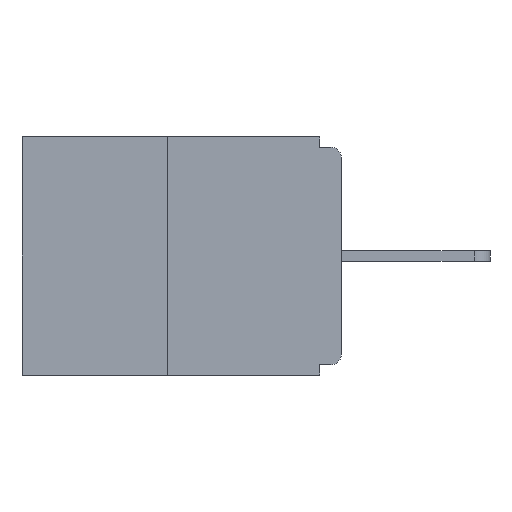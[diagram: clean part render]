
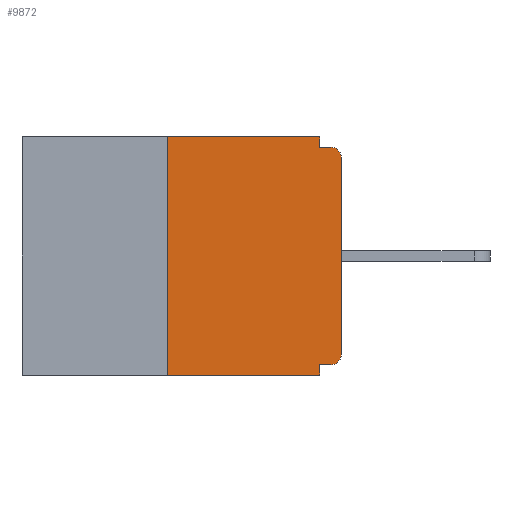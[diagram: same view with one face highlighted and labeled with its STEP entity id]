
A CAD part, left-side view. The second image highlights one B-rep face of the part: STEP entity #9872.
In plain terms, the highlighted planar face has unit normal (-1, 0, 0).
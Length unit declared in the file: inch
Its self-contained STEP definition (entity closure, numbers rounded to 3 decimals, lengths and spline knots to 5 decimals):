
#187 = ORIENTED_EDGE ( 'NONE', *, *, #12590, .F. ) ;
#594 = DIRECTION ( 'NONE',  ( -1., 0., 0. ) ) ;
#603 = CARTESIAN_POINT ( 'NONE',  ( 0., 0.46, -0.343 ) ) ;
#630 = VERTEX_POINT ( 'NONE', #15528 ) ;
#683 = CARTESIAN_POINT ( 'NONE',  ( 0., 0., -0.328 ) ) ;
#1034 = EDGE_CURVE ( 'NONE', #630, #7725, #15452, .T. ) ;
#1348 = VERTEX_POINT ( 'NONE', #3470 ) ;
#1537 = CARTESIAN_POINT ( 'NONE',  ( 0., 0.46, 0. ) ) ;
#1681 = CIRCLE ( 'NONE', #7419, 0.015 ) ;
#1764 = DIRECTION ( 'NONE',  ( 1., 0., 0. ) ) ;
#2621 = ORIENTED_EDGE ( 'NONE', *, *, #1034, .F. ) ;
#3470 = CARTESIAN_POINT ( 'NONE',  ( 0., 0.031, -0.328 ) ) ;
#3579 = EDGE_CURVE ( 'NONE', #10144, #4300, #1681, .T. ) ;
#3772 = CARTESIAN_POINT ( 'NONE',  ( 0., 0.031, 0. ) ) ;
#4054 = LINE ( 'NONE', #4904, #11728 ) ;
#4062 = FACE_OUTER_BOUND ( 'NONE', #11626, .T. ) ;
#4128 = CARTESIAN_POINT ( 'NONE',  ( 0., 0.015, -0.015 ) ) ;
#4300 = VERTEX_POINT ( 'NONE', #4128 ) ;
#4359 = ORIENTED_EDGE ( 'NONE', *, *, #11154, .F. ) ;
#4456 = EDGE_CURVE ( 'NONE', #8293, #1348, #12782, .T. ) ;
#4521 = LINE ( 'NONE', #6452, #7189 ) ;
#4662 = DIRECTION ( 'NONE',  ( 0., -1., 0. ) ) ;
#4704 = ORIENTED_EDGE ( 'NONE', *, *, #8900, .T. ) ;
#4904 = CARTESIAN_POINT ( 'NONE',  ( 0., 0.031, -0.343 ) ) ;
#4966 = VECTOR ( 'NONE', #4662, 39.37008 ) ;
#5309 = CARTESIAN_POINT ( 'NONE',  ( 0., 0.015, -0.03 ) ) ;
#6214 = VECTOR ( 'NONE', #6262, 39.37008 ) ;
#6239 = EDGE_CURVE ( 'NONE', #11302, #630, #4521, .T. ) ;
#6262 = DIRECTION ( 'NONE',  ( 0., 0., -1. ) ) ;
#6350 = DIRECTION ( 'NONE',  ( 0., -1., 0. ) ) ;
#6452 = CARTESIAN_POINT ( 'NONE',  ( 0., 0.25, 0. ) ) ;
#6777 = VECTOR ( 'NONE', #9120, 39.37008 ) ;
#7104 = AXIS2_PLACEMENT_3D ( 'NONE', #7850, #1764, #10217 ) ;
#7189 = VECTOR ( 'NONE', #10248, 39.37008 ) ;
#7201 = DIRECTION ( 'NONE',  ( 0., 0., -1. ) ) ;
#7419 = AXIS2_PLACEMENT_3D ( 'NONE', #5309, #594, #11681 ) ;
#7725 = VERTEX_POINT ( 'NONE', #11198 ) ;
#7850 = CARTESIAN_POINT ( 'NONE',  ( 0., 0.46, 0. ) ) ;
#7939 = LINE ( 'NONE', #603, #6777 ) ;
#7958 = DIRECTION ( 'NONE',  ( 0., 1., 0. ) ) ;
#7959 = DIRECTION ( 'NONE',  ( 0., 0., 1. ) ) ;
#7969 = AXIS2_PLACEMENT_3D ( 'NONE', #15626, #14510, #9713 ) ;
#8293 = VERTEX_POINT ( 'NONE', #13309 ) ;
#8313 = LINE ( 'NONE', #12856, #13828 ) ;
#8441 = EDGE_CURVE ( 'NONE', #11302, #13205, #7939, .T. ) ;
#8479 = CIRCLE ( 'NONE', #7969, 0.015 ) ;
#8500 = ORIENTED_EDGE ( 'NONE', *, *, #3579, .T. ) ;
#8900 = EDGE_CURVE ( 'NONE', #14369, #10144, #8313, .T. ) ;
#9066 = LINE ( 'NONE', #3772, #6214 ) ;
#9084 = ORIENTED_EDGE ( 'NONE', *, *, #4456, .F. ) ;
#9120 = DIRECTION ( 'NONE',  ( 0., -1., 0. ) ) ;
#9559 = CARTESIAN_POINT ( 'NONE',  ( 0., 0., -0.015 ) ) ;
#9713 = DIRECTION ( 'NONE',  ( 0., 0., -1. ) ) ;
#9872 = ADVANCED_FACE ( 'NONE', ( #4062 ), #10358, .F. ) ;
#9884 = CARTESIAN_POINT ( 'NONE',  ( 0., 0.031, -0.015 ) ) ;
#10144 = VERTEX_POINT ( 'NONE', #15000 ) ;
#10217 = DIRECTION ( 'NONE',  ( 0., 0., -1. ) ) ;
#10248 = DIRECTION ( 'NONE',  ( 0., 0., 1. ) ) ;
#10358 = PLANE ( 'NONE',  #7104 ) ;
#10647 = CARTESIAN_POINT ( 'NONE',  ( 0., 0.031, -0.343 ) ) ;
#10865 = ORIENTED_EDGE ( 'NONE', *, *, #8441, .T. ) ;
#11154 = EDGE_CURVE ( 'NONE', #11315, #4300, #15293, .T. ) ;
#11198 = CARTESIAN_POINT ( 'NONE',  ( 0., 0.031, 0. ) ) ;
#11302 = VERTEX_POINT ( 'NONE', #12170 ) ;
#11315 = VERTEX_POINT ( 'NONE', #9884 ) ;
#11484 = ORIENTED_EDGE ( 'NONE', *, *, #11630, .F. ) ;
#11626 = EDGE_LOOP ( 'NONE', ( #2621, #11956, #10865, #187, #9084, #14712, #4704, #8500, #4359, #11484 ) ) ;
#11630 = EDGE_CURVE ( 'NONE', #7725, #11315, #9066, .T. ) ;
#11681 = DIRECTION ( 'NONE',  ( 0., 0., -1. ) ) ;
#11728 = VECTOR ( 'NONE', #7201, 39.37008 ) ;
#11956 = ORIENTED_EDGE ( 'NONE', *, *, #6239, .F. ) ;
#12170 = CARTESIAN_POINT ( 'NONE',  ( 0., 0.25, -0.343 ) ) ;
#12216 = CARTESIAN_POINT ( 'NONE',  ( 0., 0., -0.313 ) ) ;
#12590 = EDGE_CURVE ( 'NONE', #1348, #13205, #4054, .T. ) ;
#12662 = EDGE_CURVE ( 'NONE', #8293, #14369, #8479, .T. ) ;
#12782 = LINE ( 'NONE', #683, #14676 ) ;
#12856 = CARTESIAN_POINT ( 'NONE',  ( 0., 0., 0. ) ) ;
#13205 = VERTEX_POINT ( 'NONE', #10647 ) ;
#13309 = CARTESIAN_POINT ( 'NONE',  ( 0., 0.015, -0.328 ) ) ;
#13828 = VECTOR ( 'NONE', #7959, 39.37008 ) ;
#14310 = VECTOR ( 'NONE', #6350, 39.37008 ) ;
#14369 = VERTEX_POINT ( 'NONE', #12216 ) ;
#14510 = DIRECTION ( 'NONE',  ( -1., 0., 0. ) ) ;
#14676 = VECTOR ( 'NONE', #7958, 39.37008 ) ;
#14712 = ORIENTED_EDGE ( 'NONE', *, *, #12662, .T. ) ;
#15000 = CARTESIAN_POINT ( 'NONE',  ( 0., 0., -0.03 ) ) ;
#15293 = LINE ( 'NONE', #9559, #4966 ) ;
#15452 = LINE ( 'NONE', #1537, #14310 ) ;
#15528 = CARTESIAN_POINT ( 'NONE',  ( 0., 0.25, 0. ) ) ;
#15626 = CARTESIAN_POINT ( 'NONE',  ( 0., 0.015, -0.313 ) ) ;
